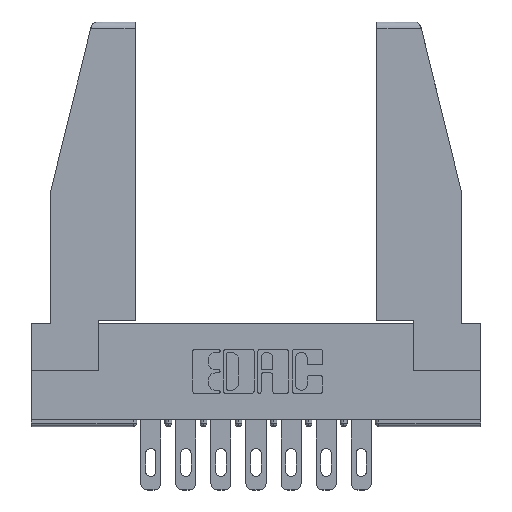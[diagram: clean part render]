
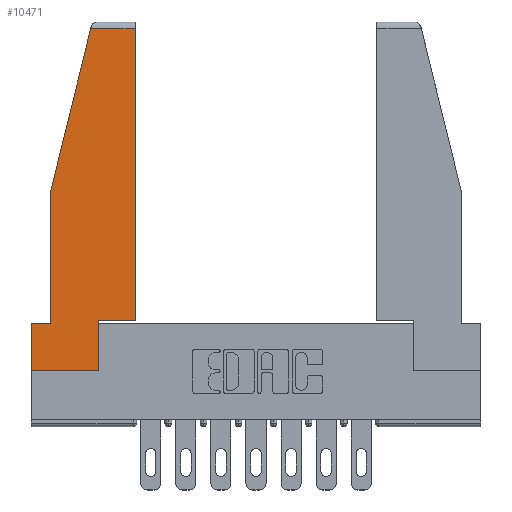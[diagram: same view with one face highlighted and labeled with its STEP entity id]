
A CAD part, top view. The second image highlights one B-rep face of the part: STEP entity #10471.
In plain terms, the highlighted planar face has unit normal (0, 0, 1).
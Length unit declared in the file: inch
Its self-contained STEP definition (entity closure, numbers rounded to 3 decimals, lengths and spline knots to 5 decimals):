
#146 = AXIS2_PLACEMENT_3D ( 'NONE', #12865, #8614, #970 ) ;
#247 = ORIENTED_EDGE ( 'NONE', *, *, #11874, .T. ) ;
#690 = ORIENTED_EDGE ( 'NONE', *, *, #10328, .T. ) ;
#795 = ORIENTED_EDGE ( 'NONE', *, *, #7629, .T. ) ;
#970 = DIRECTION ( 'NONE',  ( 1., 0., 0. ) ) ;
#1083 = FACE_OUTER_BOUND ( 'NONE', #5841, .T. ) ;
#1354 = CARTESIAN_POINT ( 'NONE',  ( 0., 1.52, 0. ) ) ;
#1368 = CARTESIAN_POINT ( 'NONE',  ( 0.086, 0.21, 0. ) ) ;
#1500 = EDGE_CURVE ( 'NONE', #12026, #6449, #6232, .T. ) ;
#1601 = CARTESIAN_POINT ( 'NONE',  ( 0.271, 1.55, 0. ) ) ;
#2399 = LINE ( 'NONE', #13009, #6386 ) ;
#2414 = CARTESIAN_POINT ( 'NONE',  ( 0.297, 0.223, 0. ) ) ;
#2501 = ORIENTED_EDGE ( 'NONE', *, *, #12109, .T. ) ;
#2865 = EDGE_CURVE ( 'NONE', #8203, #8671, #5310, .T. ) ;
#3008 = ORIENTED_EDGE ( 'NONE', *, *, #2865, .T. ) ;
#3580 = CARTESIAN_POINT ( 'NONE',  ( 0.461, 1.52, 0. ) ) ;
#4476 = CARTESIAN_POINT ( 'NONE',  ( 0.461, 0.223, 0. ) ) ;
#4586 = VERTEX_POINT ( 'NONE', #3580 ) ;
#4606 = ORIENTED_EDGE ( 'NONE', *, *, #13078, .T. ) ;
#4718 = CARTESIAN_POINT ( 'NONE',  ( 0.086, 0.8, 0. ) ) ;
#4925 = CARTESIAN_POINT ( 'NONE',  ( 0., 0., 0. ) ) ;
#4974 = VECTOR ( 'NONE', #8713, 39.37008 ) ;
#5140 = CARTESIAN_POINT ( 'NONE',  ( 0.297, 0., 0. ) ) ;
#5281 = DIRECTION ( 'NONE',  ( 0., 1., 0. ) ) ;
#5310 = LINE ( 'NONE', #5490, #4974 ) ;
#5490 = CARTESIAN_POINT ( 'NONE',  ( 0., 0.21, 0. ) ) ;
#5551 = ORIENTED_EDGE ( 'NONE', *, *, #1500, .T. ) ;
#5716 = LINE ( 'NONE', #4718, #9038 ) ;
#5841 = EDGE_LOOP ( 'NONE', ( #4606, #10404, #690, #247, #3008, #2501, #5551, #11271, #795 ) ) ;
#6040 = DIRECTION ( 'NONE',  ( -0.239, -0.971, 0. ) ) ;
#6080 = VECTOR ( 'NONE', #9157, 39.37008 ) ;
#6101 = LINE ( 'NONE', #6878, #8200 ) ;
#6201 = CARTESIAN_POINT ( 'NONE',  ( 0., 0., 0. ) ) ;
#6232 = LINE ( 'NONE', #6201, #13158 ) ;
#6386 = VECTOR ( 'NONE', #7497, 39.37008 ) ;
#6449 = VERTEX_POINT ( 'NONE', #13539 ) ;
#6686 = DIRECTION ( 'NONE',  ( 1., 0., 0. ) ) ;
#6745 = CARTESIAN_POINT ( 'NONE',  ( 0., 0.21, 0. ) ) ;
#6878 = CARTESIAN_POINT ( 'NONE',  ( 0.297, 0.223, 0. ) ) ;
#6909 = VERTEX_POINT ( 'NONE', #13770 ) ;
#6953 = LINE ( 'NONE', #1354, #6080 ) ;
#7436 = DIRECTION ( 'NONE',  ( 0., -1., 0. ) ) ;
#7497 = DIRECTION ( 'NONE',  ( 0., 1., 0. ) ) ;
#7629 = EDGE_CURVE ( 'NONE', #13318, #11829, #6101, .T. ) ;
#7816 = VECTOR ( 'NONE', #5281, 39.37008 ) ;
#8106 = DIRECTION ( 'NONE',  ( 0., -1., 0. ) ) ;
#8200 = VECTOR ( 'NONE', #6686, 39.37008 ) ;
#8203 = VERTEX_POINT ( 'NONE', #1368 ) ;
#8543 = LINE ( 'NONE', #1601, #8896 ) ;
#8575 = EDGE_CURVE ( 'NONE', #6449, #13318, #13531, .T. ) ;
#8614 = DIRECTION ( 'NONE',  ( 0., 0., 1. ) ) ;
#8671 = VERTEX_POINT ( 'NONE', #6745 ) ;
#8713 = DIRECTION ( 'NONE',  ( -1., 0., 0. ) ) ;
#8896 = VECTOR ( 'NONE', #6040, 39.37008 ) ;
#9038 = VECTOR ( 'NONE', #8106, 39.37008 ) ;
#9157 = DIRECTION ( 'NONE',  ( -1., 0., 0. ) ) ;
#10228 = VERTEX_POINT ( 'NONE', #10333 ) ;
#10328 = EDGE_CURVE ( 'NONE', #6909, #10228, #8543, .T. ) ;
#10333 = CARTESIAN_POINT ( 'NONE',  ( 0.086, 0.8, 0. ) ) ;
#10404 = ORIENTED_EDGE ( 'NONE', *, *, #11609, .T. ) ;
#10471 = ADVANCED_FACE ( 'NONE', ( #1083 ), #10664, .T. ) ;
#10664 = PLANE ( 'NONE',  #146 ) ;
#10808 = CARTESIAN_POINT ( 'NONE',  ( 0., 0.21, 0. ) ) ;
#11271 = ORIENTED_EDGE ( 'NONE', *, *, #8575, .T. ) ;
#11609 = EDGE_CURVE ( 'NONE', #4586, #6909, #6953, .T. ) ;
#11773 = DIRECTION ( 'NONE',  ( 1., 0., 0. ) ) ;
#11829 = VERTEX_POINT ( 'NONE', #4476 ) ;
#11874 = EDGE_CURVE ( 'NONE', #10228, #8203, #5716, .T. ) ;
#12026 = VERTEX_POINT ( 'NONE', #4925 ) ;
#12109 = EDGE_CURVE ( 'NONE', #8671, #12026, #12987, .T. ) ;
#12865 = CARTESIAN_POINT ( 'NONE',  ( 0., 0., 0. ) ) ;
#12987 = LINE ( 'NONE', #10808, #13508 ) ;
#13009 = CARTESIAN_POINT ( 'NONE',  ( 0.461, 0.223, 0. ) ) ;
#13078 = EDGE_CURVE ( 'NONE', #11829, #4586, #2399, .T. ) ;
#13158 = VECTOR ( 'NONE', #11773, 39.37008 ) ;
#13318 = VERTEX_POINT ( 'NONE', #2414 ) ;
#13508 = VECTOR ( 'NONE', #7436, 39.37008 ) ;
#13531 = LINE ( 'NONE', #5140, #7816 ) ;
#13539 = CARTESIAN_POINT ( 'NONE',  ( 0.297, 0., 0. ) ) ;
#13770 = CARTESIAN_POINT ( 'NONE',  ( 0.2636, 1.52, 0. ) ) ;
